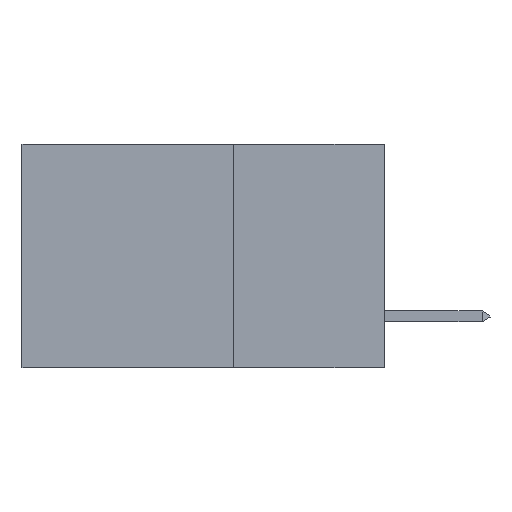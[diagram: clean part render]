
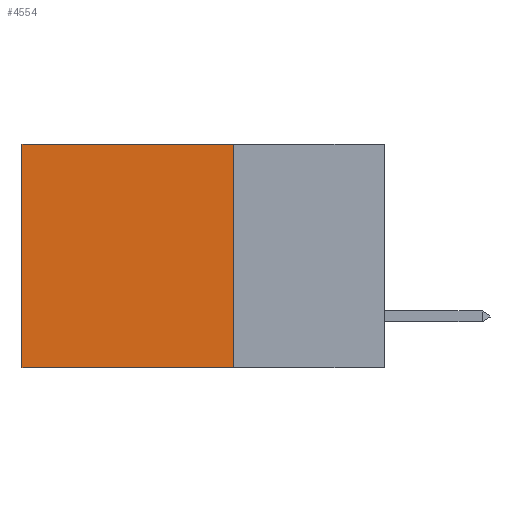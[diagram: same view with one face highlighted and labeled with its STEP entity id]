
A CAD part, left-side view. The second image highlights one B-rep face of the part: STEP entity #4554.
In plain terms, the highlighted planar face has unit normal (-1, 0, 0).
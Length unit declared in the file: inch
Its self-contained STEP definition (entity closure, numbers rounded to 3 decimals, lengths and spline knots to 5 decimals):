
#138 = VERTEX_POINT ( 'NONE', #17465 ) ;
#416 = CARTESIAN_POINT ( 'NONE',  ( 0.2875, 0.25, 0. ) ) ;
#714 = VECTOR ( 'NONE', #14110, 39.37008 ) ;
#1002 = CARTESIAN_POINT ( 'NONE',  ( 0.2875, 0.25, 0. ) ) ;
#1044 = VERTEX_POINT ( 'NONE', #11017 ) ;
#1359 = ORIENTED_EDGE ( 'NONE', *, *, #16172, .T. ) ;
#1497 = EDGE_LOOP ( 'NONE', ( #18353, #18738, #14943, #1359 ) ) ;
#2079 = LINE ( 'NONE', #21370, #3680 ) ;
#3680 = VECTOR ( 'NONE', #16255, 39.37008 ) ;
#4070 = LINE ( 'NONE', #1002, #21458 ) ;
#4479 = DIRECTION ( 'NONE',  ( 0., 0., -1. ) ) ;
#4554 = ADVANCED_FACE ( 'NONE', ( #13301 ), #6838, .F. ) ;
#5055 = DIRECTION ( 'NONE',  ( 1., 0., 0. ) ) ;
#5102 = VERTEX_POINT ( 'NONE', #19872 ) ;
#5137 = DIRECTION ( 'NONE',  ( 0., 0., -1. ) ) ;
#6838 = PLANE ( 'NONE',  #21780 ) ;
#8299 = EDGE_CURVE ( 'NONE', #1044, #138, #2079, .T. ) ;
#8318 = CARTESIAN_POINT ( 'NONE',  ( 0.2875, 0.25, 0. ) ) ;
#9530 = VERTEX_POINT ( 'NONE', #10005 ) ;
#10005 = CARTESIAN_POINT ( 'NONE',  ( 0.2875, 0.25, -0.37 ) ) ;
#11017 = CARTESIAN_POINT ( 'NONE',  ( 0.2875, 0.6, 0. ) ) ;
#11061 = LINE ( 'NONE', #416, #714 ) ;
#11245 = VECTOR ( 'NONE', #12279, 39.37008 ) ;
#11484 = EDGE_CURVE ( 'NONE', #9530, #138, #14153, .T. ) ;
#12279 = DIRECTION ( 'NONE',  ( 0., 1., 0. ) ) ;
#13301 = FACE_OUTER_BOUND ( 'NONE', #1497, .T. ) ;
#14110 = DIRECTION ( 'NONE',  ( 0., 1., 0. ) ) ;
#14153 = LINE ( 'NONE', #15404, #11245 ) ;
#14943 = ORIENTED_EDGE ( 'NONE', *, *, #18082, .F. ) ;
#15404 = CARTESIAN_POINT ( 'NONE',  ( 0.2875, 0.25, -0.37 ) ) ;
#16172 = EDGE_CURVE ( 'NONE', #5102, #1044, #11061, .T. ) ;
#16255 = DIRECTION ( 'NONE',  ( 0., 0., -1. ) ) ;
#17465 = CARTESIAN_POINT ( 'NONE',  ( 0.2875, 0.6, -0.37 ) ) ;
#18082 = EDGE_CURVE ( 'NONE', #5102, #9530, #4070, .T. ) ;
#18353 = ORIENTED_EDGE ( 'NONE', *, *, #8299, .T. ) ;
#18738 = ORIENTED_EDGE ( 'NONE', *, *, #11484, .F. ) ;
#19872 = CARTESIAN_POINT ( 'NONE',  ( 0.2875, 0.25, 0. ) ) ;
#21370 = CARTESIAN_POINT ( 'NONE',  ( 0.2875, 0.6, 0. ) ) ;
#21458 = VECTOR ( 'NONE', #4479, 39.37008 ) ;
#21780 = AXIS2_PLACEMENT_3D ( 'NONE', #8318, #5055, #5137 ) ;
